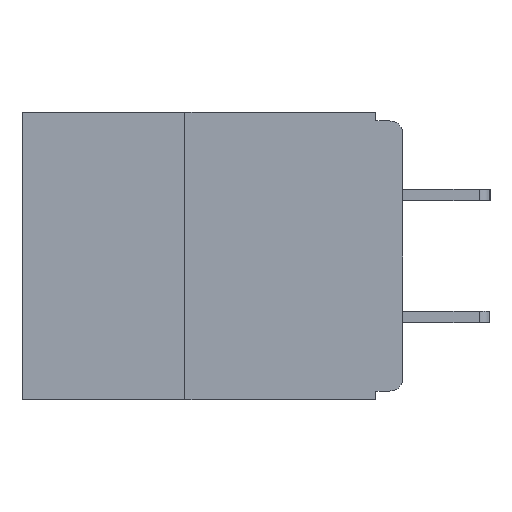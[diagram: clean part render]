
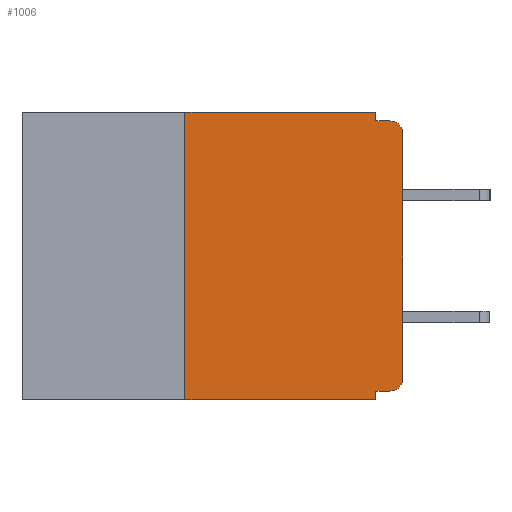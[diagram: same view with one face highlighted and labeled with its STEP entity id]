
A CAD part, left-side view. The second image highlights one B-rep face of the part: STEP entity #1006.
In plain terms, the highlighted planar face has unit normal (-1, 0, 0).
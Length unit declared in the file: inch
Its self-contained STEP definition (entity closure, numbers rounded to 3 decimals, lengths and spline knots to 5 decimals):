
#29 = ORIENTED_EDGE ( 'NONE', *, *, #29133, .F. ) ;
#73 = VECTOR ( 'NONE', #11478, 39.37008 ) ;
#301 = DIRECTION ( 'NONE',  ( 0., 0., -1. ) ) ;
#1006 = ADVANCED_FACE ( 'NONE', ( #17551 ), #28141, .F. ) ;
#2141 = VERTEX_POINT ( 'NONE', #19750 ) ;
#2475 = ORIENTED_EDGE ( 'NONE', *, *, #29044, .F. ) ;
#2519 = CARTESIAN_POINT ( 'NONE',  ( 0., 0.437, 0. ) ) ;
#2541 = EDGE_CURVE ( 'NONE', #9152, #26136, #11379, .T. ) ;
#2681 = ORIENTED_EDGE ( 'NONE', *, *, #9307, .T. ) ;
#3030 = DIRECTION ( 'NONE',  ( 0., -1., 0. ) ) ;
#3252 = ORIENTED_EDGE ( 'NONE', *, *, #26770, .F. ) ;
#4255 = LINE ( 'NONE', #6906, #16479 ) ;
#4429 = DIRECTION ( 'NONE',  ( 0., 0., -1. ) ) ;
#4992 = CARTESIAN_POINT ( 'NONE',  ( 0., 0.031, 0. ) ) ;
#5205 = AXIS2_PLACEMENT_3D ( 'NONE', #29525, #31477, #30766 ) ;
#5754 = VECTOR ( 'NONE', #23990, 39.37008 ) ;
#5899 = CARTESIAN_POINT ( 'NONE',  ( 0., 0.015, -0.025 ) ) ;
#6577 = EDGE_CURVE ( 'NONE', #26136, #30753, #29545, .T. ) ;
#6906 = CARTESIAN_POINT ( 'NONE',  ( 0., 0.25, -0.33 ) ) ;
#8290 = DIRECTION ( 'NONE',  ( 0., 0., -1. ) ) ;
#8773 = VERTEX_POINT ( 'NONE', #23283 ) ;
#9152 = VERTEX_POINT ( 'NONE', #12153 ) ;
#9182 = CARTESIAN_POINT ( 'NONE',  ( 0., 0.031, -0.32 ) ) ;
#9225 = CARTESIAN_POINT ( 'NONE',  ( 0., 0., -0.32 ) ) ;
#9307 = EDGE_CURVE ( 'NONE', #10910, #18119, #14517, .T. ) ;
#9820 = CARTESIAN_POINT ( 'NONE',  ( 0., 0.031, 0. ) ) ;
#9837 = VERTEX_POINT ( 'NONE', #29200 ) ;
#9884 = VECTOR ( 'NONE', #24352, 39.37008 ) ;
#10020 = VECTOR ( 'NONE', #4429, 39.37008 ) ;
#10910 = VERTEX_POINT ( 'NONE', #14256 ) ;
#11379 = LINE ( 'NONE', #2519, #12151 ) ;
#11478 = DIRECTION ( 'NONE',  ( 0., 0., -1. ) ) ;
#11684 = EDGE_CURVE ( 'NONE', #9837, #20776, #19836, .T. ) ;
#11788 = DIRECTION ( 'NONE',  ( 0., 0., 1. ) ) ;
#11918 = ORIENTED_EDGE ( 'NONE', *, *, #6577, .F. ) ;
#12151 = VECTOR ( 'NONE', #3030, 39.37008 ) ;
#12153 = CARTESIAN_POINT ( 'NONE',  ( 0., 0.25, 0. ) ) ;
#12197 = LINE ( 'NONE', #9225, #5754 ) ;
#13223 = LINE ( 'NONE', #24524, #25557 ) ;
#13289 = VECTOR ( 'NONE', #16309, 39.37008 ) ;
#14256 = CARTESIAN_POINT ( 'NONE',  ( 0., 0., -0.025 ) ) ;
#14517 = CIRCLE ( 'NONE', #28174, 0.015 ) ;
#14614 = DIRECTION ( 'NONE',  ( 0., -1., 0. ) ) ;
#14865 = DIRECTION ( 'NONE',  ( -1., 0., 0. ) ) ;
#15800 = ORIENTED_EDGE ( 'NONE', *, *, #20272, .T. ) ;
#16155 = AXIS2_PLACEMENT_3D ( 'NONE', #29506, #14865, #301 ) ;
#16309 = DIRECTION ( 'NONE',  ( 0., -1., 0. ) ) ;
#16479 = VECTOR ( 'NONE', #11788, 39.37008 ) ;
#17246 = LINE ( 'NONE', #19452, #9884 ) ;
#17551 = FACE_OUTER_BOUND ( 'NONE', #18640, .T. ) ;
#18119 = VERTEX_POINT ( 'NONE', #21481 ) ;
#18640 = EDGE_LOOP ( 'NONE', ( #18737, #2681, #3252, #11918, #29191, #29, #15800, #2475, #22838, #30100 ) ) ;
#18737 = ORIENTED_EDGE ( 'NONE', *, *, #24277, .T. ) ;
#19452 = CARTESIAN_POINT ( 'NONE',  ( 0., 0., 0. ) ) ;
#19593 = LINE ( 'NONE', #21310, #73 ) ;
#19750 = CARTESIAN_POINT ( 'NONE',  ( 0., 0.25, -0.33 ) ) ;
#19836 = CIRCLE ( 'NONE', #16155, 0.015 ) ;
#19882 = VERTEX_POINT ( 'NONE', #9182 ) ;
#20272 = EDGE_CURVE ( 'NONE', #2141, #8773, #26365, .T. ) ;
#20697 = CARTESIAN_POINT ( 'NONE',  ( 0., 0., -0.305 ) ) ;
#20776 = VERTEX_POINT ( 'NONE', #20697 ) ;
#21163 = CARTESIAN_POINT ( 'NONE',  ( 0., 0.437, -0.33 ) ) ;
#21310 = CARTESIAN_POINT ( 'NONE',  ( 0., 0.031, -0.33 ) ) ;
#21481 = CARTESIAN_POINT ( 'NONE',  ( 0., 0.015, -0.01 ) ) ;
#22673 = CARTESIAN_POINT ( 'NONE',  ( 0., 0.031, -0.01 ) ) ;
#22838 = ORIENTED_EDGE ( 'NONE', *, *, #24850, .F. ) ;
#23048 = DIRECTION ( 'NONE',  ( -1., 0., 0. ) ) ;
#23283 = CARTESIAN_POINT ( 'NONE',  ( 0., 0.031, -0.33 ) ) ;
#23990 = DIRECTION ( 'NONE',  ( 0., 1., 0. ) ) ;
#24277 = EDGE_CURVE ( 'NONE', #20776, #10910, #17246, .T. ) ;
#24352 = DIRECTION ( 'NONE',  ( 0., 0., 1. ) ) ;
#24524 = CARTESIAN_POINT ( 'NONE',  ( 0., 0., -0.01 ) ) ;
#24850 = EDGE_CURVE ( 'NONE', #9837, #19882, #12197, .T. ) ;
#25557 = VECTOR ( 'NONE', #14614, 39.37008 ) ;
#26136 = VERTEX_POINT ( 'NONE', #9820 ) ;
#26365 = LINE ( 'NONE', #21163, #13289 ) ;
#26770 = EDGE_CURVE ( 'NONE', #30753, #18119, #13223, .T. ) ;
#28141 = PLANE ( 'NONE',  #5205 ) ;
#28174 = AXIS2_PLACEMENT_3D ( 'NONE', #5899, #23048, #8290 ) ;
#29044 = EDGE_CURVE ( 'NONE', #19882, #8773, #19593, .T. ) ;
#29133 = EDGE_CURVE ( 'NONE', #2141, #9152, #4255, .T. ) ;
#29191 = ORIENTED_EDGE ( 'NONE', *, *, #2541, .F. ) ;
#29200 = CARTESIAN_POINT ( 'NONE',  ( 0., 0.015, -0.32 ) ) ;
#29506 = CARTESIAN_POINT ( 'NONE',  ( 0., 0.015, -0.305 ) ) ;
#29525 = CARTESIAN_POINT ( 'NONE',  ( 0., 0.437, 0. ) ) ;
#29545 = LINE ( 'NONE', #4992, #10020 ) ;
#30100 = ORIENTED_EDGE ( 'NONE', *, *, #11684, .T. ) ;
#30753 = VERTEX_POINT ( 'NONE', #22673 ) ;
#30766 = DIRECTION ( 'NONE',  ( 0., 0., -1. ) ) ;
#31477 = DIRECTION ( 'NONE',  ( 1., 0., 0. ) ) ;
